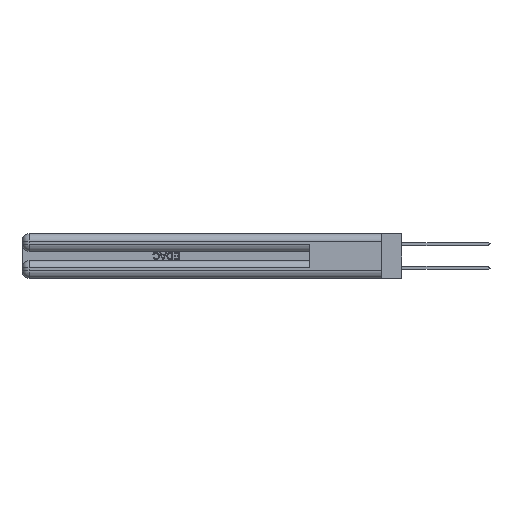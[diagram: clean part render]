
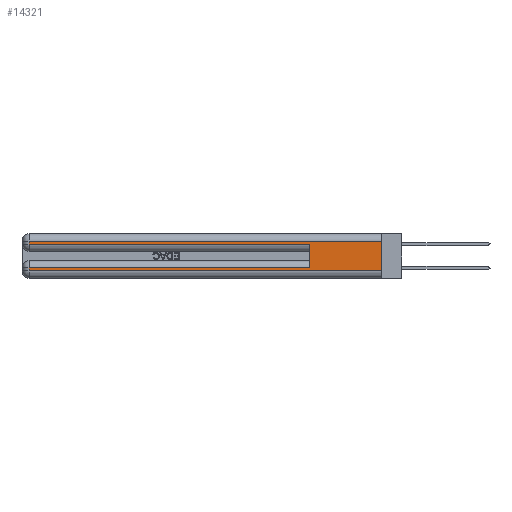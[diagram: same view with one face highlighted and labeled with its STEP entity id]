
A CAD part, left-side view. The second image highlights one B-rep face of the part: STEP entity #14321.
In plain terms, the highlighted planar face has unit normal (-1, 0, 0).
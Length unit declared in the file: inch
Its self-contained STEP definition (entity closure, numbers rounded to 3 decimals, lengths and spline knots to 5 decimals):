
#451 = DIRECTION ( 'NONE',  ( 0., 0., -1. ) ) ;
#2143 = DIRECTION ( 'NONE',  ( 0., 0., -1. ) ) ;
#2657 = VERTEX_POINT ( 'NONE', #20836 ) ;
#3009 = VERTEX_POINT ( 'NONE', #5374 ) ;
#3265 = VERTEX_POINT ( 'NONE', #21627 ) ;
#5374 = CARTESIAN_POINT ( 'NONE',  ( 0., 0.6, 0.285 ) ) ;
#5779 = CARTESIAN_POINT ( 'NONE',  ( 0., 2.94, 0.37 ) ) ;
#5822 = CARTESIAN_POINT ( 'NONE',  ( 0., 0.6, 0.145 ) ) ;
#6279 = ORIENTED_EDGE ( 'NONE', *, *, #33402, .T. ) ;
#6909 = EDGE_CURVE ( 'NONE', #38176, #34083, #13396, .T. ) ;
#7119 = LINE ( 'NONE', #8165, #31018 ) ;
#7303 = VECTOR ( 'NONE', #15847, 39.37008 ) ;
#8165 = CARTESIAN_POINT ( 'NONE',  ( 0., 0., 0.31 ) ) ;
#9002 = DIRECTION ( 'NONE',  ( 0., 0., 1. ) ) ;
#9726 = EDGE_CURVE ( 'NONE', #10863, #38176, #7119, .T. ) ;
#9972 = VERTEX_POINT ( 'NONE', #14766 ) ;
#10750 = VECTOR ( 'NONE', #24838, 39.37008 ) ;
#10863 = VERTEX_POINT ( 'NONE', #27849 ) ;
#12804 = CARTESIAN_POINT ( 'NONE',  ( 0., 0.6, 0.085 ) ) ;
#12922 = FACE_OUTER_BOUND ( 'NONE', #29061, .T. ) ;
#13396 = LINE ( 'NONE', #32253, #39267 ) ;
#14321 = ADVANCED_FACE ( 'NONE', ( #12922 ), #18774, .F. ) ;
#14766 = CARTESIAN_POINT ( 'NONE',  ( 0., 0., 0.06 ) ) ;
#15183 = CARTESIAN_POINT ( 'NONE',  ( 0., 0., 0.285 ) ) ;
#15233 = AXIS2_PLACEMENT_3D ( 'NONE', #18633, #21993, #2143 ) ;
#15847 = DIRECTION ( 'NONE',  ( 0., 0., -1. ) ) ;
#16329 = ORIENTED_EDGE ( 'NONE', *, *, #9726, .T. ) ;
#16571 = LINE ( 'NONE', #5822, #18676 ) ;
#16844 = CARTESIAN_POINT ( 'NONE',  ( 0., 0., 0.37 ) ) ;
#17476 = ORIENTED_EDGE ( 'NONE', *, *, #32710, .T. ) ;
#18061 = DIRECTION ( 'NONE',  ( 0., 0., -1. ) ) ;
#18365 = CARTESIAN_POINT ( 'NONE',  ( 0., 2.94, 0.285 ) ) ;
#18633 = CARTESIAN_POINT ( 'NONE',  ( 0., 0., 0.37 ) ) ;
#18676 = VECTOR ( 'NONE', #9002, 39.37008 ) ;
#18774 = PLANE ( 'NONE',  #15233 ) ;
#19563 = LINE ( 'NONE', #31832, #10750 ) ;
#19843 = ORIENTED_EDGE ( 'NONE', *, *, #6909, .T. ) ;
#20762 = EDGE_CURVE ( 'NONE', #2657, #9972, #28515, .T. ) ;
#20836 = CARTESIAN_POINT ( 'NONE',  ( 0., 2.94, 0.06 ) ) ;
#21627 = CARTESIAN_POINT ( 'NONE',  ( 0., 2.94, 0.085 ) ) ;
#21652 = DIRECTION ( 'NONE',  ( 0., 1., 0. ) ) ;
#21993 = DIRECTION ( 'NONE',  ( 1., 0., 0. ) ) ;
#24838 = DIRECTION ( 'NONE',  ( 0., 1., 0. ) ) ;
#25203 = DIRECTION ( 'NONE',  ( 0., -1., 0. ) ) ;
#25348 = DIRECTION ( 'NONE',  ( 0., -1., 0. ) ) ;
#25740 = LINE ( 'NONE', #15183, #33503 ) ;
#25915 = ORIENTED_EDGE ( 'NONE', *, *, #20762, .T. ) ;
#27849 = CARTESIAN_POINT ( 'NONE',  ( 0., 0., 0.31 ) ) ;
#28004 = CARTESIAN_POINT ( 'NONE',  ( 0., 0., 0.06 ) ) ;
#28075 = LINE ( 'NONE', #5779, #7303 ) ;
#28515 = LINE ( 'NONE', #28004, #35208 ) ;
#28571 = VERTEX_POINT ( 'NONE', #12804 ) ;
#29061 = EDGE_LOOP ( 'NONE', ( #42596, #16329, #19843, #6279, #34765, #17476, #33846, #25915 ) ) ;
#30012 = EDGE_CURVE ( 'NONE', #3265, #2657, #28075, .T. ) ;
#30271 = EDGE_CURVE ( 'NONE', #10863, #9972, #42506, .T. ) ;
#30541 = EDGE_CURVE ( 'NONE', #28571, #3009, #16571, .T. ) ;
#31018 = VECTOR ( 'NONE', #21652, 39.37008 ) ;
#31701 = VECTOR ( 'NONE', #451, 39.37008 ) ;
#31832 = CARTESIAN_POINT ( 'NONE',  ( 0., 0., 0.085 ) ) ;
#32253 = CARTESIAN_POINT ( 'NONE',  ( 0., 2.94, 0.37 ) ) ;
#32710 = EDGE_CURVE ( 'NONE', #28571, #3265, #19563, .T. ) ;
#32800 = CARTESIAN_POINT ( 'NONE',  ( 0., 2.94, 0.31 ) ) ;
#33402 = EDGE_CURVE ( 'NONE', #34083, #3009, #25740, .T. ) ;
#33503 = VECTOR ( 'NONE', #25203, 39.37008 ) ;
#33846 = ORIENTED_EDGE ( 'NONE', *, *, #30012, .T. ) ;
#34083 = VERTEX_POINT ( 'NONE', #18365 ) ;
#34765 = ORIENTED_EDGE ( 'NONE', *, *, #30541, .F. ) ;
#35208 = VECTOR ( 'NONE', #25348, 39.37008 ) ;
#38176 = VERTEX_POINT ( 'NONE', #32800 ) ;
#39267 = VECTOR ( 'NONE', #18061, 39.37008 ) ;
#42506 = LINE ( 'NONE', #16844, #31701 ) ;
#42596 = ORIENTED_EDGE ( 'NONE', *, *, #30271, .F. ) ;
